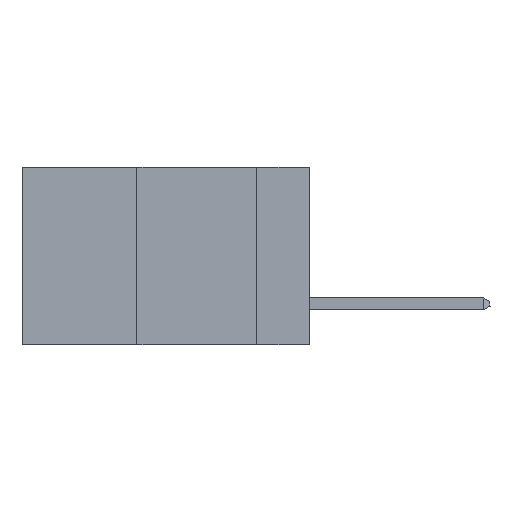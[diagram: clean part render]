
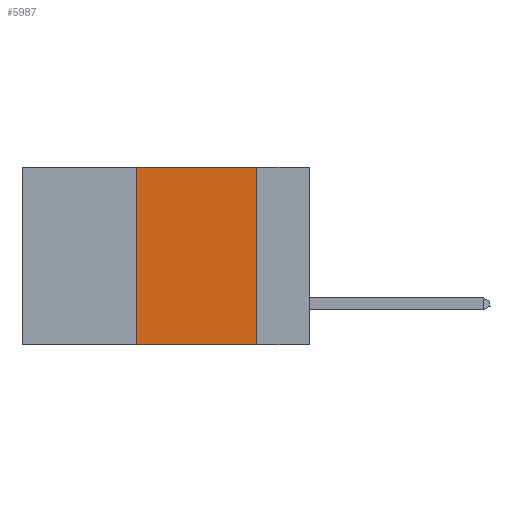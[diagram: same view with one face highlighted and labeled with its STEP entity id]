
A CAD part, left-side view. The second image highlights one B-rep face of the part: STEP entity #5987.
In plain terms, the highlighted planar face has unit normal (-1, 0, 0).
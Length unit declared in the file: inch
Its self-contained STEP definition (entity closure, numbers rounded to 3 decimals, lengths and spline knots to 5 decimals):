
#580 = VECTOR ( 'NONE', #10712, 39.37008 ) ;
#799 = ORIENTED_EDGE ( 'NONE', *, *, #8275, .F. ) ;
#1066 = LINE ( 'NONE', #12211, #5906 ) ;
#1651 = DIRECTION ( 'NONE',  ( 0., 0., -1. ) ) ;
#1740 = VECTOR ( 'NONE', #7404, 39.37008 ) ;
#2409 = EDGE_CURVE ( 'NONE', #4041, #8822, #1066, .T. ) ;
#2626 = VERTEX_POINT ( 'NONE', #3747 ) ;
#2996 = CARTESIAN_POINT ( 'NONE',  ( 0., 0.6, 0. ) ) ;
#3112 = CARTESIAN_POINT ( 'NONE',  ( 0., 0.11, 0. ) ) ;
#3414 = DIRECTION ( 'NONE',  ( 0., -1., 0. ) ) ;
#3747 = CARTESIAN_POINT ( 'NONE',  ( 0., 0.36, 0. ) ) ;
#4041 = VERTEX_POINT ( 'NONE', #6980 ) ;
#4350 = CARTESIAN_POINT ( 'NONE',  ( 0., 0.36, 0. ) ) ;
#4761 = ORIENTED_EDGE ( 'NONE', *, *, #6030, .F. ) ;
#4944 = VERTEX_POINT ( 'NONE', #3112 ) ;
#5340 = VECTOR ( 'NONE', #12183, 39.37008 ) ;
#5411 = ORIENTED_EDGE ( 'NONE', *, *, #2409, .T. ) ;
#5500 = DIRECTION ( 'NONE',  ( 1., 0., 0. ) ) ;
#5671 = CARTESIAN_POINT ( 'NONE',  ( 0., 0.6, 0. ) ) ;
#5906 = VECTOR ( 'NONE', #3414, 39.37008 ) ;
#5987 = ADVANCED_FACE ( 'NONE', ( #12420 ), #6499, .F. ) ;
#6030 = EDGE_CURVE ( 'NONE', #2626, #4944, #8338, .T. ) ;
#6094 = LINE ( 'NONE', #4350, #5340 ) ;
#6499 = PLANE ( 'NONE',  #11334 ) ;
#6574 = ORIENTED_EDGE ( 'NONE', *, *, #11499, .F. ) ;
#6575 = CARTESIAN_POINT ( 'NONE',  ( 0., 0.11, 0. ) ) ;
#6980 = CARTESIAN_POINT ( 'NONE',  ( 0., 0.36, -0.37 ) ) ;
#7404 = DIRECTION ( 'NONE',  ( 0., 0., -1. ) ) ;
#8275 = EDGE_CURVE ( 'NONE', #4944, #8822, #8861, .T. ) ;
#8338 = LINE ( 'NONE', #2996, #580 ) ;
#8822 = VERTEX_POINT ( 'NONE', #10182 ) ;
#8861 = LINE ( 'NONE', #6575, #1740 ) ;
#10182 = CARTESIAN_POINT ( 'NONE',  ( 0., 0.11, -0.37 ) ) ;
#10712 = DIRECTION ( 'NONE',  ( 0., -1., 0. ) ) ;
#11334 = AXIS2_PLACEMENT_3D ( 'NONE', #5671, #5500, #1651 ) ;
#11499 = EDGE_CURVE ( 'NONE', #4041, #2626, #6094, .T. ) ;
#11716 = EDGE_LOOP ( 'NONE', ( #799, #4761, #6574, #5411 ) ) ;
#12183 = DIRECTION ( 'NONE',  ( 0., 0., 1. ) ) ;
#12211 = CARTESIAN_POINT ( 'NONE',  ( 0., 0.6, -0.37 ) ) ;
#12420 = FACE_OUTER_BOUND ( 'NONE', #11716, .T. ) ;
